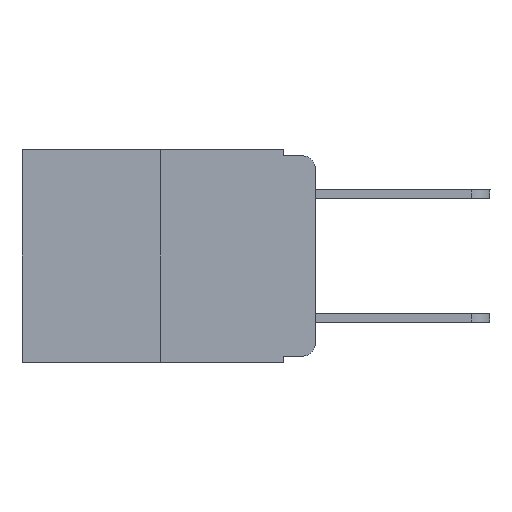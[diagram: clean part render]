
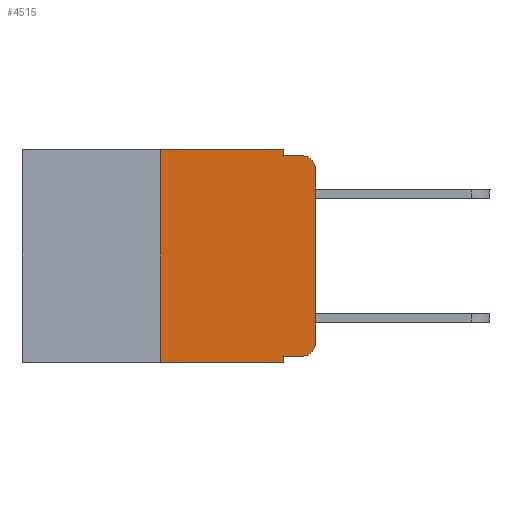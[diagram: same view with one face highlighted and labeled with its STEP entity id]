
A CAD part, left-side view. The second image highlights one B-rep face of the part: STEP entity #4515.
In plain terms, the highlighted planar face has unit normal (-1, 0, 0).
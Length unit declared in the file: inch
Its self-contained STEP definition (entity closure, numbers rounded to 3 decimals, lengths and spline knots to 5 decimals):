
#676 = AXIS2_PLACEMENT_3D ( 'NONE', #18495, #8626, #16988 ) ;
#760 = CARTESIAN_POINT ( 'NONE',  ( 0., 0., -0.313 ) ) ;
#1478 = LINE ( 'NONE', #14500, #3007 ) ;
#2380 = DIRECTION ( 'NONE',  ( 0., -1., 0. ) ) ;
#2957 = DIRECTION ( 'NONE',  ( 0., 0., -1. ) ) ;
#3007 = VECTOR ( 'NONE', #15357, 39.37008 ) ;
#3105 = DIRECTION ( 'NONE',  ( 0., -1., 0. ) ) ;
#3506 = VECTOR ( 'NONE', #7749, 39.37008 ) ;
#3511 = CARTESIAN_POINT ( 'NONE',  ( 0., 0.051, -0.343 ) ) ;
#3649 = CARTESIAN_POINT ( 'NONE',  ( 0., 0.051, -0.01 ) ) ;
#3759 = CARTESIAN_POINT ( 'NONE',  ( 0., 0.02, -0.03 ) ) ;
#4173 = CARTESIAN_POINT ( 'NONE',  ( 0., 0.25, -0.343 ) ) ;
#4217 = FACE_OUTER_BOUND ( 'NONE', #9014, .T. ) ;
#4461 = EDGE_CURVE ( 'NONE', #13778, #4582, #1478, .T. ) ;
#4515 = ADVANCED_FACE ( 'NONE', ( #4217 ), #14309, .F. ) ;
#4516 = CARTESIAN_POINT ( 'NONE',  ( 0., 0.051, -0.333 ) ) ;
#4561 = VECTOR ( 'NONE', #10483, 39.37008 ) ;
#4582 = VERTEX_POINT ( 'NONE', #14596 ) ;
#4597 = ORIENTED_EDGE ( 'NONE', *, *, #10923, .T. ) ;
#4778 = ORIENTED_EDGE ( 'NONE', *, *, #12557, .F. ) ;
#4826 = LINE ( 'NONE', #10405, #3506 ) ;
#4945 = ORIENTED_EDGE ( 'NONE', *, *, #10945, .F. ) ;
#5456 = VERTEX_POINT ( 'NONE', #8965 ) ;
#5662 = EDGE_CURVE ( 'NONE', #5456, #7379, #12986, .T. ) ;
#5697 = LINE ( 'NONE', #12680, #8827 ) ;
#5872 = VERTEX_POINT ( 'NONE', #8665 ) ;
#5894 = VERTEX_POINT ( 'NONE', #10365 ) ;
#6325 = CARTESIAN_POINT ( 'NONE',  ( 0., 0., 0. ) ) ;
#7020 = VERTEX_POINT ( 'NONE', #760 ) ;
#7379 = VERTEX_POINT ( 'NONE', #13643 ) ;
#7749 = DIRECTION ( 'NONE',  ( 0., -1., 0. ) ) ;
#8626 = DIRECTION ( 'NONE',  ( -1., 0., 0. ) ) ;
#8665 = CARTESIAN_POINT ( 'NONE',  ( 0., 0.051, 0. ) ) ;
#8738 = AXIS2_PLACEMENT_3D ( 'NONE', #11578, #17203, #18525 ) ;
#8827 = VECTOR ( 'NONE', #2957, 39.37008 ) ;
#8940 = VERTEX_POINT ( 'NONE', #3649 ) ;
#8965 = CARTESIAN_POINT ( 'NONE',  ( 0., 0., -0.03 ) ) ;
#9014 = EDGE_LOOP ( 'NONE', ( #10057, #11377, #10120, #4945, #18059, #12192, #9339, #4778, #11915, #4597 ) ) ;
#9161 = LINE ( 'NONE', #6325, #4561 ) ;
#9339 = ORIENTED_EDGE ( 'NONE', *, *, #11130, .T. ) ;
#9629 = EDGE_CURVE ( 'NONE', #7020, #5456, #9161, .T. ) ;
#9725 = CARTESIAN_POINT ( 'NONE',  ( 0., 0.473, 0. ) ) ;
#9779 = EDGE_CURVE ( 'NONE', #4582, #5872, #18358, .T. ) ;
#9945 = EDGE_CURVE ( 'NONE', #15316, #5894, #9993, .T. ) ;
#9993 = LINE ( 'NONE', #4516, #11511 ) ;
#10057 = ORIENTED_EDGE ( 'NONE', *, *, #9629, .T. ) ;
#10120 = ORIENTED_EDGE ( 'NONE', *, *, #16667, .F. ) ;
#10365 = CARTESIAN_POINT ( 'NONE',  ( 0., 0.02, -0.333 ) ) ;
#10405 = CARTESIAN_POINT ( 'NONE',  ( 0., 0.051, -0.01 ) ) ;
#10483 = DIRECTION ( 'NONE',  ( 0., 0., 1. ) ) ;
#10923 = EDGE_CURVE ( 'NONE', #5894, #7020, #11538, .T. ) ;
#10943 = DIRECTION ( 'NONE',  ( 0., -1., 0. ) ) ;
#10945 = EDGE_CURVE ( 'NONE', #5872, #8940, #5697, .T. ) ;
#11130 = EDGE_CURVE ( 'NONE', #13778, #12286, #17347, .T. ) ;
#11224 = DIRECTION ( 'NONE',  ( 0., 0., -1. ) ) ;
#11377 = ORIENTED_EDGE ( 'NONE', *, *, #5662, .T. ) ;
#11487 = VECTOR ( 'NONE', #10943, 39.37008 ) ;
#11511 = VECTOR ( 'NONE', #3105, 39.37008 ) ;
#11538 = CIRCLE ( 'NONE', #676, 0.02 ) ;
#11578 = CARTESIAN_POINT ( 'NONE',  ( 0., 0.473, 0. ) ) ;
#11832 = VECTOR ( 'NONE', #12944, 39.37008 ) ;
#11915 = ORIENTED_EDGE ( 'NONE', *, *, #9945, .T. ) ;
#12158 = CARTESIAN_POINT ( 'NONE',  ( 0., 0.051, -0.333 ) ) ;
#12191 = CARTESIAN_POINT ( 'NONE',  ( 0., 0.473, -0.343 ) ) ;
#12192 = ORIENTED_EDGE ( 'NONE', *, *, #4461, .F. ) ;
#12286 = VERTEX_POINT ( 'NONE', #3511 ) ;
#12528 = DIRECTION ( 'NONE',  ( -1., 0., 0. ) ) ;
#12557 = EDGE_CURVE ( 'NONE', #15316, #12286, #12663, .T. ) ;
#12663 = LINE ( 'NONE', #14446, #11832 ) ;
#12680 = CARTESIAN_POINT ( 'NONE',  ( 0., 0.051, 0. ) ) ;
#12944 = DIRECTION ( 'NONE',  ( 0., 0., -1. ) ) ;
#12986 = CIRCLE ( 'NONE', #14489, 0.02 ) ;
#13032 = VECTOR ( 'NONE', #2380, 39.37008 ) ;
#13643 = CARTESIAN_POINT ( 'NONE',  ( 0., 0.02, -0.01 ) ) ;
#13778 = VERTEX_POINT ( 'NONE', #4173 ) ;
#14309 = PLANE ( 'NONE',  #8738 ) ;
#14446 = CARTESIAN_POINT ( 'NONE',  ( 0., 0.051, 0. ) ) ;
#14489 = AXIS2_PLACEMENT_3D ( 'NONE', #3759, #12528, #11224 ) ;
#14500 = CARTESIAN_POINT ( 'NONE',  ( 0., 0.25, 0. ) ) ;
#14596 = CARTESIAN_POINT ( 'NONE',  ( 0., 0.25, 0. ) ) ;
#15316 = VERTEX_POINT ( 'NONE', #12158 ) ;
#15357 = DIRECTION ( 'NONE',  ( 0., 0., 1. ) ) ;
#16667 = EDGE_CURVE ( 'NONE', #8940, #7379, #4826, .T. ) ;
#16988 = DIRECTION ( 'NONE',  ( 0., 0., -1. ) ) ;
#17203 = DIRECTION ( 'NONE',  ( 1., 0., 0. ) ) ;
#17347 = LINE ( 'NONE', #12191, #13032 ) ;
#18059 = ORIENTED_EDGE ( 'NONE', *, *, #9779, .F. ) ;
#18358 = LINE ( 'NONE', #9725, #11487 ) ;
#18495 = CARTESIAN_POINT ( 'NONE',  ( 0., 0.02, -0.313 ) ) ;
#18525 = DIRECTION ( 'NONE',  ( 0., 0., -1. ) ) ;
